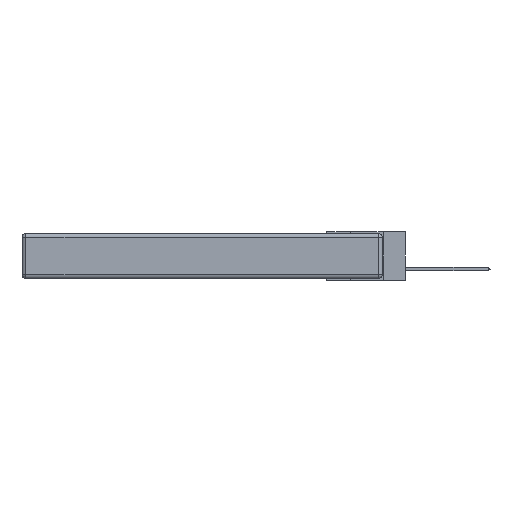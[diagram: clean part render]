
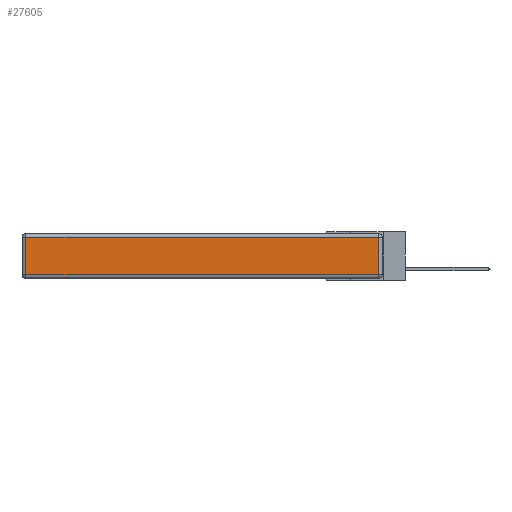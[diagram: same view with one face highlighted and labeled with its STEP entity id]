
A CAD part, left-side view. The second image highlights one B-rep face of the part: STEP entity #27605.
In plain terms, the highlighted planar face has unit normal (-1, 0, 0).
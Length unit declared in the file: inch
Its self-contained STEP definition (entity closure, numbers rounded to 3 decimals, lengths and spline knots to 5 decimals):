
#314 = CARTESIAN_POINT ( 'NONE',  ( 0., 2.72, -0.313 ) ) ;
#1451 = DIRECTION ( 'NONE',  ( 0., 0., 1. ) ) ;
#4738 = LINE ( 'NONE', #24996, #18626 ) ;
#5046 = CARTESIAN_POINT ( 'NONE',  ( 0., 0., -0.343 ) ) ;
#5596 = EDGE_CURVE ( 'NONE', #8383, #17657, #5690, .T. ) ;
#5609 = VECTOR ( 'NONE', #1451, 39.37008 ) ;
#5631 = EDGE_LOOP ( 'NONE', ( #29221, #14530, #17768, #14992 ) ) ;
#5690 = LINE ( 'NONE', #20111, #17896 ) ;
#6609 = FACE_OUTER_BOUND ( 'NONE', #5631, .T. ) ;
#8383 = VERTEX_POINT ( 'NONE', #8763 ) ;
#8763 = CARTESIAN_POINT ( 'NONE',  ( 0., 0.03, -0.03 ) ) ;
#8978 = LINE ( 'NONE', #9207, #5609 ) ;
#9207 = CARTESIAN_POINT ( 'NONE',  ( 0., 0.03, -0.343 ) ) ;
#9543 = DIRECTION ( 'NONE',  ( 0., 1., 0. ) ) ;
#10804 = PLANE ( 'NONE',  #29868 ) ;
#14530 = ORIENTED_EDGE ( 'NONE', *, *, #23946, .T. ) ;
#14992 = ORIENTED_EDGE ( 'NONE', *, *, #33722, .T. ) ;
#16077 = DIRECTION ( 'NONE',  ( 0., 0., 1. ) ) ;
#16873 = DIRECTION ( 'NONE',  ( 0., -1., 0. ) ) ;
#17657 = VERTEX_POINT ( 'NONE', #18488 ) ;
#17768 = ORIENTED_EDGE ( 'NONE', *, *, #5596, .T. ) ;
#17896 = VECTOR ( 'NONE', #9543, 39.37008 ) ;
#18488 = CARTESIAN_POINT ( 'NONE',  ( 0., 2.72, -0.03 ) ) ;
#18626 = VECTOR ( 'NONE', #16873, 39.37008 ) ;
#19078 = VERTEX_POINT ( 'NONE', #24506 ) ;
#19352 = VECTOR ( 'NONE', #32441, 39.37008 ) ;
#20111 = CARTESIAN_POINT ( 'NONE',  ( 0., 2.75, -0.03 ) ) ;
#23946 = EDGE_CURVE ( 'NONE', #19078, #8383, #8978, .T. ) ;
#24506 = CARTESIAN_POINT ( 'NONE',  ( 0., 0.03, -0.313 ) ) ;
#24878 = EDGE_CURVE ( 'NONE', #32446, #19078, #4738, .T. ) ;
#24996 = CARTESIAN_POINT ( 'NONE',  ( 0., 0., -0.313 ) ) ;
#27605 = ADVANCED_FACE ( 'NONE', ( #6609 ), #10804, .T. ) ;
#29221 = ORIENTED_EDGE ( 'NONE', *, *, #24878, .T. ) ;
#29686 = CARTESIAN_POINT ( 'NONE',  ( 0., 2.72, -0.343 ) ) ;
#29868 = AXIS2_PLACEMENT_3D ( 'NONE', #5046, #32103, #16077 ) ;
#32103 = DIRECTION ( 'NONE',  ( -1., 0., 0. ) ) ;
#32441 = DIRECTION ( 'NONE',  ( 0., 0., -1. ) ) ;
#32446 = VERTEX_POINT ( 'NONE', #314 ) ;
#32710 = LINE ( 'NONE', #29686, #19352 ) ;
#33722 = EDGE_CURVE ( 'NONE', #17657, #32446, #32710, .T. ) ;
